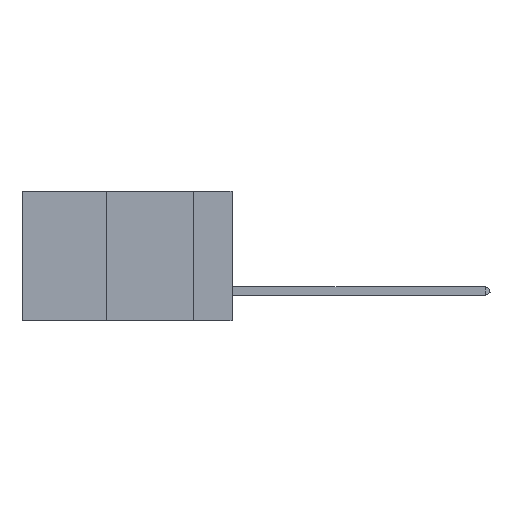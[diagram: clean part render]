
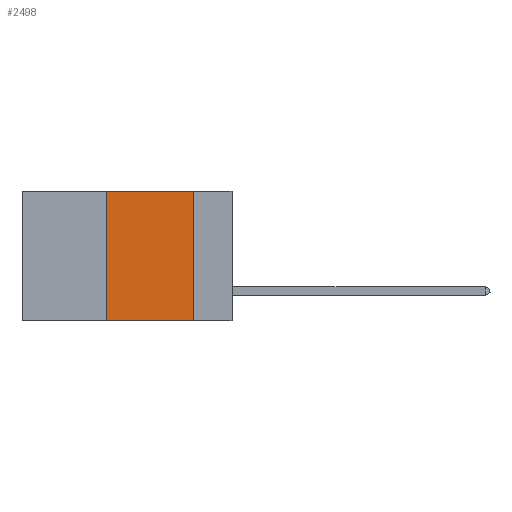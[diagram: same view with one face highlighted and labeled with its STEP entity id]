
A CAD part, left-side view. The second image highlights one B-rep face of the part: STEP entity #2498.
In plain terms, the highlighted planar face has unit normal (-1, 0, 0).
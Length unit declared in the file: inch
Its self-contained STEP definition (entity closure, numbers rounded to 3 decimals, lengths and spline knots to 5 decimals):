
#764 = CARTESIAN_POINT ( 'NONE',  ( 0., 0.6, 0. ) ) ;
#784 = VECTOR ( 'NONE', #4931, 39.37008 ) ;
#1198 = CARTESIAN_POINT ( 'NONE',  ( 0., 0.36, 0. ) ) ;
#1402 = PLANE ( 'NONE',  #2924 ) ;
#1438 = DIRECTION ( 'NONE',  ( 1., 0., 0. ) ) ;
#1473 = LINE ( 'NONE', #6144, #2737 ) ;
#1745 = CARTESIAN_POINT ( 'NONE',  ( 0., 0.11, -0.37 ) ) ;
#1944 = EDGE_CURVE ( 'NONE', #3951, #1999, #7691, .T. ) ;
#1999 = VERTEX_POINT ( 'NONE', #3223 ) ;
#2240 = DIRECTION ( 'NONE',  ( 0., 0., -1. ) ) ;
#2287 = LINE ( 'NONE', #3895, #6338 ) ;
#2498 = ADVANCED_FACE ( 'NONE', ( #4316 ), #1402, .F. ) ;
#2737 = VECTOR ( 'NONE', #6979, 39.37008 ) ;
#2924 = AXIS2_PLACEMENT_3D ( 'NONE', #5480, #1438, #2240 ) ;
#2977 = EDGE_CURVE ( 'NONE', #3835, #10186, #5305, .T. ) ;
#3045 = ORIENTED_EDGE ( 'NONE', *, *, #6619, .F. ) ;
#3223 = CARTESIAN_POINT ( 'NONE',  ( 0., 0.11, 0. ) ) ;
#3308 = CARTESIAN_POINT ( 'NONE',  ( 0., 0.6, -0.37 ) ) ;
#3835 = VERTEX_POINT ( 'NONE', #6913 ) ;
#3889 = ORIENTED_EDGE ( 'NONE', *, *, #2977, .T. ) ;
#3895 = CARTESIAN_POINT ( 'NONE',  ( 0., 0.11, 0. ) ) ;
#3951 = VERTEX_POINT ( 'NONE', #1198 ) ;
#4316 = FACE_OUTER_BOUND ( 'NONE', #7951, .T. ) ;
#4619 = EDGE_CURVE ( 'NONE', #1999, #10186, #2287, .T. ) ;
#4702 = DIRECTION ( 'NONE',  ( 0., -1., 0. ) ) ;
#4931 = DIRECTION ( 'NONE',  ( 0., -1., 0. ) ) ;
#5305 = LINE ( 'NONE', #3308, #784 ) ;
#5480 = CARTESIAN_POINT ( 'NONE',  ( 0., 0.6, 0. ) ) ;
#5750 = ORIENTED_EDGE ( 'NONE', *, *, #4619, .F. ) ;
#6144 = CARTESIAN_POINT ( 'NONE',  ( 0., 0.36, 0. ) ) ;
#6338 = VECTOR ( 'NONE', #10541, 39.37008 ) ;
#6619 = EDGE_CURVE ( 'NONE', #3835, #3951, #1473, .T. ) ;
#6913 = CARTESIAN_POINT ( 'NONE',  ( 0., 0.36, -0.37 ) ) ;
#6979 = DIRECTION ( 'NONE',  ( 0., 0., 1. ) ) ;
#7691 = LINE ( 'NONE', #764, #10307 ) ;
#7792 = ORIENTED_EDGE ( 'NONE', *, *, #1944, .F. ) ;
#7951 = EDGE_LOOP ( 'NONE', ( #5750, #7792, #3045, #3889 ) ) ;
#10186 = VERTEX_POINT ( 'NONE', #1745 ) ;
#10307 = VECTOR ( 'NONE', #4702, 39.37008 ) ;
#10541 = DIRECTION ( 'NONE',  ( 0., 0., -1. ) ) ;
